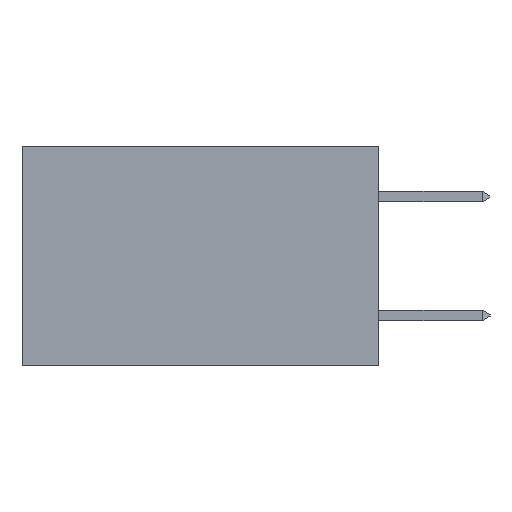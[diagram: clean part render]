
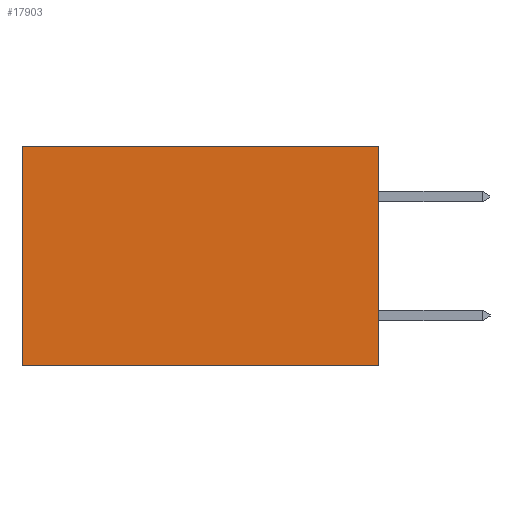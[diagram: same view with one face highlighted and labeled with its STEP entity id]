
A CAD part, left-side view. The second image highlights one B-rep face of the part: STEP entity #17903.
In plain terms, the highlighted planar face has unit normal (-1, 0, 0).
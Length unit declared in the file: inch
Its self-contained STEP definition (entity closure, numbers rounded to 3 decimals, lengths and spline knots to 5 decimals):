
#333 = DIRECTION ( 'NONE',  ( 0., 1., 0. ) ) ;
#357 = CARTESIAN_POINT ( 'NONE',  ( 0.2615, 0., -0.37 ) ) ;
#361 = VECTOR ( 'NONE', #2612, 39.37008 ) ;
#1090 = CARTESIAN_POINT ( 'NONE',  ( 0.2615, 0., -0.37 ) ) ;
#1532 = CARTESIAN_POINT ( 'NONE',  ( 0.2615, 0.6, -0.37 ) ) ;
#2107 = VERTEX_POINT ( 'NONE', #14908 ) ;
#2612 = DIRECTION ( 'NONE',  ( 0., 0., -1. ) ) ;
#2787 = FACE_OUTER_BOUND ( 'NONE', #14812, .T. ) ;
#3981 = LINE ( 'NONE', #357, #11707 ) ;
#4216 = CARTESIAN_POINT ( 'NONE',  ( 0.2615, 0., -0.37 ) ) ;
#5091 = PLANE ( 'NONE',  #8159 ) ;
#5119 = CARTESIAN_POINT ( 'NONE',  ( 0.2615, 0.6, 0. ) ) ;
#5628 = EDGE_CURVE ( 'NONE', #11042, #11506, #17635, .T. ) ;
#6285 = VECTOR ( 'NONE', #16090, 39.37008 ) ;
#6576 = DIRECTION ( 'NONE',  ( 1., 0., 0. ) ) ;
#7357 = VERTEX_POINT ( 'NONE', #4216 ) ;
#8159 = AXIS2_PLACEMENT_3D ( 'NONE', #12300, #6576, #16558 ) ;
#8659 = EDGE_CURVE ( 'NONE', #7357, #2107, #3981, .T. ) ;
#8745 = ORIENTED_EDGE ( 'NONE', *, *, #12509, .T. ) ;
#11042 = VERTEX_POINT ( 'NONE', #11412 ) ;
#11412 = CARTESIAN_POINT ( 'NONE',  ( 0.2615, 0., 0. ) ) ;
#11506 = VERTEX_POINT ( 'NONE', #5119 ) ;
#11689 = EDGE_CURVE ( 'NONE', #11042, #7357, #12012, .T. ) ;
#11707 = VECTOR ( 'NONE', #333, 39.37008 ) ;
#11725 = DIRECTION ( 'NONE',  ( 0., 0., -1. ) ) ;
#12012 = LINE ( 'NONE', #1090, #361 ) ;
#12300 = CARTESIAN_POINT ( 'NONE',  ( 0.2615, 0., -0.37 ) ) ;
#12509 = EDGE_CURVE ( 'NONE', #11506, #2107, #13621, .T. ) ;
#12842 = ORIENTED_EDGE ( 'NONE', *, *, #8659, .F. ) ;
#13180 = VECTOR ( 'NONE', #11725, 39.37008 ) ;
#13621 = LINE ( 'NONE', #1532, #13180 ) ;
#14812 = EDGE_LOOP ( 'NONE', ( #8745, #12842, #15582, #15381 ) ) ;
#14908 = CARTESIAN_POINT ( 'NONE',  ( 0.2615, 0.6, -0.37 ) ) ;
#15381 = ORIENTED_EDGE ( 'NONE', *, *, #5628, .T. ) ;
#15582 = ORIENTED_EDGE ( 'NONE', *, *, #11689, .F. ) ;
#15930 = CARTESIAN_POINT ( 'NONE',  ( 0.2615, 0., 0. ) ) ;
#16090 = DIRECTION ( 'NONE',  ( 0., 1., 0. ) ) ;
#16558 = DIRECTION ( 'NONE',  ( 0., 0., -1. ) ) ;
#17635 = LINE ( 'NONE', #15930, #6285 ) ;
#17903 = ADVANCED_FACE ( 'NONE', ( #2787 ), #5091, .F. ) ;
